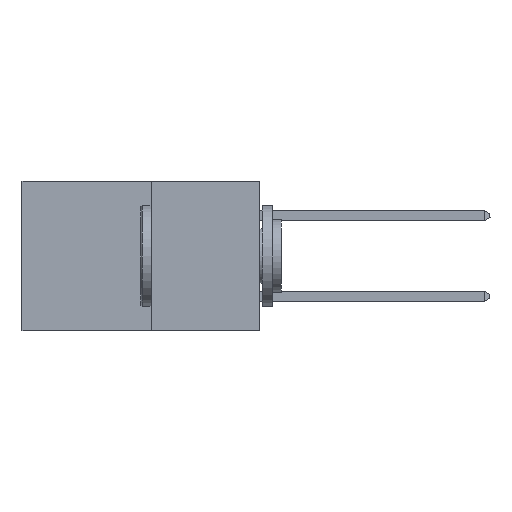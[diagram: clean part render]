
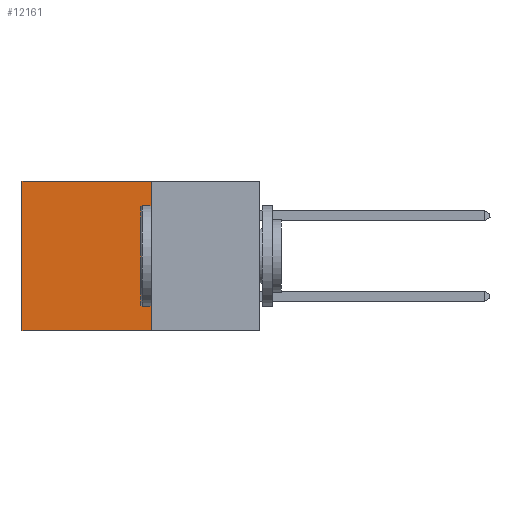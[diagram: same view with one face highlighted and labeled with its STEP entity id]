
A CAD part, left-side view. The second image highlights one B-rep face of the part: STEP entity #12161.
In plain terms, the highlighted planar face has unit normal (-1, 0, 0).
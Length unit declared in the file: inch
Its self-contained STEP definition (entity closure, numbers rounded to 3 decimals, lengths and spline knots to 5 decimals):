
#486 = CARTESIAN_POINT ( 'NONE',  ( 0.277, 0.27, 0. ) ) ;
#1297 = AXIS2_PLACEMENT_3D ( 'NONE', #17412, #3414, #13212 ) ;
#1837 = CARTESIAN_POINT ( 'NONE',  ( 0.277, 0.59, -0.37 ) ) ;
#1929 = EDGE_CURVE ( 'NONE', #7262, #11410, #2247, .T. ) ;
#1942 = DIRECTION ( 'NONE',  ( 0., 1., 0. ) ) ;
#1949 = PLANE ( 'NONE',  #1297 ) ;
#1976 = ORIENTED_EDGE ( 'NONE', *, *, #1929, .F. ) ;
#2022 = CARTESIAN_POINT ( 'NONE',  ( 0.277, 0.59, 0. ) ) ;
#2247 = LINE ( 'NONE', #6141, #9776 ) ;
#3077 = EDGE_CURVE ( 'NONE', #12825, #7262, #16995, .T. ) ;
#3299 = ORIENTED_EDGE ( 'NONE', *, *, #3077, .F. ) ;
#3414 = DIRECTION ( 'NONE',  ( 1., 0., 0. ) ) ;
#3440 = CARTESIAN_POINT ( 'NONE',  ( 0.277, 0.27, 0. ) ) ;
#3944 = LINE ( 'NONE', #17660, #7670 ) ;
#4573 = ORIENTED_EDGE ( 'NONE', *, *, #9352, .T. ) ;
#5497 = EDGE_CURVE ( 'NONE', #9552, #11410, #3944, .T. ) ;
#6141 = CARTESIAN_POINT ( 'NONE',  ( 0.277, 0.27, -0.37 ) ) ;
#6221 = VECTOR ( 'NONE', #16411, 39.37008 ) ;
#6278 = DIRECTION ( 'NONE',  ( 0., 1., 0. ) ) ;
#7262 = VERTEX_POINT ( 'NONE', #15595 ) ;
#7359 = VECTOR ( 'NONE', #1942, 39.37008 ) ;
#7670 = VECTOR ( 'NONE', #14832, 39.37008 ) ;
#9231 = FACE_OUTER_BOUND ( 'NONE', #13865, .T. ) ;
#9352 = EDGE_CURVE ( 'NONE', #12825, #9552, #11525, .T. ) ;
#9552 = VERTEX_POINT ( 'NONE', #2022 ) ;
#9776 = VECTOR ( 'NONE', #6278, 39.37008 ) ;
#11410 = VERTEX_POINT ( 'NONE', #1837 ) ;
#11525 = LINE ( 'NONE', #486, #7359 ) ;
#12161 = ADVANCED_FACE ( 'NONE', ( #9231 ), #1949, .F. ) ;
#12825 = VERTEX_POINT ( 'NONE', #3440 ) ;
#13212 = DIRECTION ( 'NONE',  ( 0., 0., -1. ) ) ;
#13718 = ORIENTED_EDGE ( 'NONE', *, *, #5497, .T. ) ;
#13865 = EDGE_LOOP ( 'NONE', ( #13718, #1976, #3299, #4573 ) ) ;
#14832 = DIRECTION ( 'NONE',  ( 0., 0., -1. ) ) ;
#15595 = CARTESIAN_POINT ( 'NONE',  ( 0.277, 0.27, -0.37 ) ) ;
#16411 = DIRECTION ( 'NONE',  ( 0., 0., -1. ) ) ;
#16432 = CARTESIAN_POINT ( 'NONE',  ( 0.277, 0.27, -0.37 ) ) ;
#16995 = LINE ( 'NONE', #16432, #6221 ) ;
#17412 = CARTESIAN_POINT ( 'NONE',  ( 0.277, 0.27, -0.37 ) ) ;
#17660 = CARTESIAN_POINT ( 'NONE',  ( 0.277, 0.59, -0.37 ) ) ;
